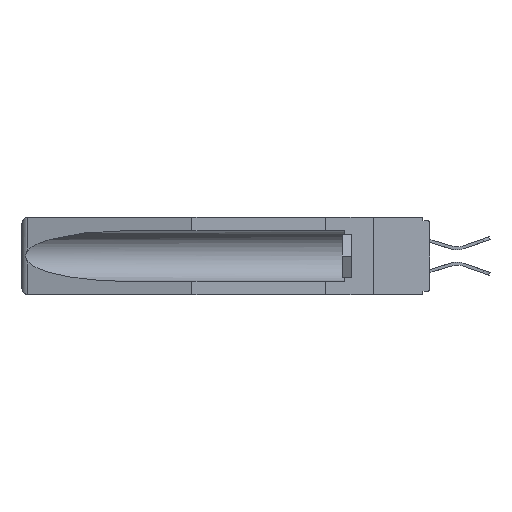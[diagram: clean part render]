
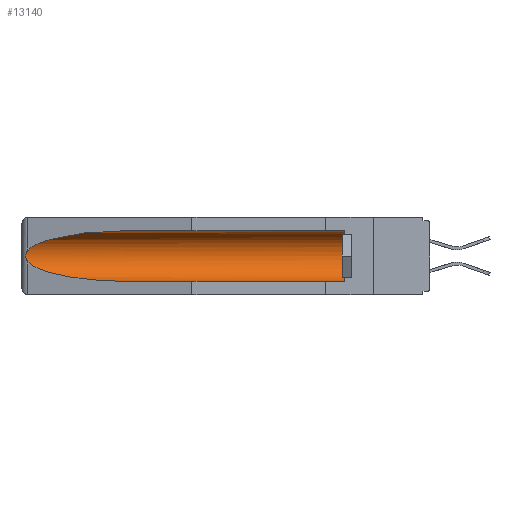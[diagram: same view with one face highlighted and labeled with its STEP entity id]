
A CAD part, left-side view. The second image highlights one B-rep face of the part: STEP entity #13140.
In plain terms, the highlighted cylindrical face has radius 2.857 mm (diameter 5.715 mm), a partial arc.
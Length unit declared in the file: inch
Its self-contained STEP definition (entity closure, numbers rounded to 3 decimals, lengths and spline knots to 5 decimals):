
#982 = CARTESIAN_POINT ( 'NONE',  ( 0.155, 0.126, -0.284 ) ) ;
#1077 = EDGE_CURVE ( 'NONE', #20654, #24298, #17854, .T. ) ;
#2189 = CARTESIAN_POINT ( 'NONE',  ( 0.26654, 1.53092, -0.15636 ) ) ;
#2275 = DIRECTION ( 'NONE',  ( 0., 1., 0. ) ) ;
#2573 = DIRECTION ( 'NONE',  ( 0., -1., 0. ) ) ;
#2598 = CARTESIAN_POINT ( 'NONE',  ( 0.21114, 1.30732, -0.059 ) ) ;
#3630 = VERTEX_POINT ( 'NONE', #24077 ) ;
#4554 = CARTESIAN_POINT ( 'NONE',  ( 0.26655, 1.53094, -0.18657 ) ) ;
#5495 = VECTOR ( 'NONE', #25924, 39.37008 ) ;
#5728 = CARTESIAN_POINT ( 'NONE',  ( 0.26537, 1.52718, -0.14972 ) ) ;
#5948 = CIRCLE ( 'NONE', #32330, 0.1125 ) ;
#7113 = VERTEX_POINT ( 'NONE', #21661 ) ;
#7120 = CARTESIAN_POINT ( 'NONE',  ( 0.26597, 1.5296, -0.19026 ) ) ;
#7348 = CARTESIAN_POINT ( 'NONE',  ( 0.2673, 1.5327, -0.16383 ) ) ;
#7696 = CARTESIAN_POINT ( 'NONE',  ( 0.26537, 1.52718, -0.14972 ) ) ;
#7921 = CARTESIAN_POINT ( 'NONE',  ( 0.26537, 1.52718, -0.19328 ) ) ;
#9160 = DIRECTION ( 'NONE',  ( 0., 0., 1. ) ) ;
#9496 = CARTESIAN_POINT ( 'NONE',  ( 0.155, -0.30754, -0.1715 ) ) ;
#10659 = CARTESIAN_POINT ( 'NONE',  ( 0.155, 1.07973, -0.059 ) ) ;
#10728 = CARTESIAN_POINT ( 'NONE',  ( 0.155, 0.126, -0.059 ) ) ;
#10791 = CARTESIAN_POINT ( 'NONE',  ( 0.155, -0.30754, -0.059 ) ) ;
#10923 = EDGE_CURVE ( 'NONE', #7113, #20654, #21928, .T. ) ;
#11860 = ORIENTED_EDGE ( 'NONE', *, *, #1077, .T. ) ;
#11925 = CARTESIAN_POINT ( 'NONE',  ( 0.21114, 1.30732, -0.284 ) ) ;
#12782 = ORIENTED_EDGE ( 'NONE', *, *, #19546, .F. ) ;
#12818 = CARTESIAN_POINT ( 'NONE',  ( 0.155, -0.30754, -0.284 ) ) ;
#13140 = ADVANCED_FACE ( 'NONE', ( #15223 ), #15642, .F. ) ;
#13519 = EDGE_CURVE ( 'NONE', #32543, #18882, #5948, .T. ) ;
#14295 = AXIS2_PLACEMENT_3D ( 'NONE', #9496, #29655, #9160 ) ;
#15223 = FACE_OUTER_BOUND ( 'NONE', #27445, .T. ) ;
#15326 = CARTESIAN_POINT ( 'NONE',  ( 0.2675, 1.53308, -0.16763 ) ) ;
#15642 = CYLINDRICAL_SURFACE ( 'NONE', #14295, 0.1125 ) ;
#17365 = CARTESIAN_POINT ( 'NONE',  ( 0.2673, 1.53269, -0.17917 ) ) ;
#17854 = B_SPLINE_CURVE_WITH_KNOTS ( 'NONE', 3,
 ( #27730, #28063, #2189, #7348, #15326, #20144, #17365, #4554, #7120, #27615 ),
 .UNSPECIFIED., .F., .F.,
 ( 4, 2, 2, 2, 4 ),
 ( 0., 0.00029, 0.00058, 0.00087, 0.00117 ),
 .UNSPECIFIED. ) ;
#18301 = VECTOR ( 'NONE', #2275, 39.37008 ) ;
#18882 = VERTEX_POINT ( 'NONE', #10728 ) ;
#19280 = CARTESIAN_POINT ( 'NONE',  ( 0.26537, 1.52718, -0.19328 ) ) ;
#19546 = EDGE_CURVE ( 'NONE', #32543, #3630, #29905, .T. ) ;
#20144 = CARTESIAN_POINT ( 'NONE',  ( 0.2675, 1.53308, -0.17534 ) ) ;
#20485 =( BOUNDED_CURVE ( )  B_SPLINE_CURVE ( 3, ( #19280, #29088, #11925, #24388 ),
 .UNSPECIFIED., .F., .T. ) 
 B_SPLINE_CURVE_WITH_KNOTS ( ( 4, 4 ),
 ( 0.1948, 1.5708 ),
 .UNSPECIFIED. ) 
 CURVE ( )  GEOMETRIC_REPRESENTATION_ITEM ( )  RATIONAL_B_SPLINE_CURVE ( ( 1., 0.848, 0.848, 1. ) ) 
 REPRESENTATION_ITEM ( '' )  );
#20536 = DIRECTION ( 'NONE',  ( 0., 0., 1. ) ) ;
#20654 = VERTEX_POINT ( 'NONE', #7696 ) ;
#20873 = ORIENTED_EDGE ( 'NONE', *, *, #33185, .T. ) ;
#21661 = CARTESIAN_POINT ( 'NONE',  ( 0.155, 1.07973, -0.059 ) ) ;
#21928 =( BOUNDED_CURVE ( )  B_SPLINE_CURVE ( 3, ( #10659, #2598, #31166, #5728 ),
 .UNSPECIFIED., .F., .F. ) 
 B_SPLINE_CURVE_WITH_KNOTS ( ( 4, 4 ),
 ( 4.71239, 6.08839 ),
 .UNSPECIFIED. ) 
 CURVE ( )  GEOMETRIC_REPRESENTATION_ITEM ( )  RATIONAL_B_SPLINE_CURVE ( ( 1., 0.848, 0.848, 1. ) ) 
 REPRESENTATION_ITEM ( '' )  );
#24077 = CARTESIAN_POINT ( 'NONE',  ( 0.155, 1.07973, -0.284 ) ) ;
#24168 = ORIENTED_EDGE ( 'NONE', *, *, #13519, .T. ) ;
#24298 = VERTEX_POINT ( 'NONE', #7921 ) ;
#24388 = CARTESIAN_POINT ( 'NONE',  ( 0.155, 1.07973, -0.284 ) ) ;
#25924 = DIRECTION ( 'NONE',  ( 0., 1., 0. ) ) ;
#27288 = EDGE_CURVE ( 'NONE', #24298, #3630, #20485, .T. ) ;
#27445 = EDGE_LOOP ( 'NONE', ( #29351, #11860, #32790, #12782, #24168, #20873 ) ) ;
#27615 = CARTESIAN_POINT ( 'NONE',  ( 0.26537, 1.52718, -0.19328 ) ) ;
#27730 = CARTESIAN_POINT ( 'NONE',  ( 0.26537, 1.52718, -0.14972 ) ) ;
#28063 = CARTESIAN_POINT ( 'NONE',  ( 0.26597, 1.52961, -0.15275 ) ) ;
#29088 = CARTESIAN_POINT ( 'NONE',  ( 0.25451, 1.48313, -0.24835 ) ) ;
#29351 = ORIENTED_EDGE ( 'NONE', *, *, #10923, .T. ) ;
#29655 = DIRECTION ( 'NONE',  ( 0., 1., 0. ) ) ;
#29905 = LINE ( 'NONE', #12818, #18301 ) ;
#29984 = LINE ( 'NONE', #10791, #5495 ) ;
#30384 = CARTESIAN_POINT ( 'NONE',  ( 0.155, 0.126, -0.1715 ) ) ;
#31166 = CARTESIAN_POINT ( 'NONE',  ( 0.25451, 1.48313, -0.09465 ) ) ;
#32330 = AXIS2_PLACEMENT_3D ( 'NONE', #30384, #2573, #20536 ) ;
#32543 = VERTEX_POINT ( 'NONE', #982 ) ;
#32790 = ORIENTED_EDGE ( 'NONE', *, *, #27288, .T. ) ;
#33185 = EDGE_CURVE ( 'NONE', #18882, #7113, #29984, .T. ) ;
